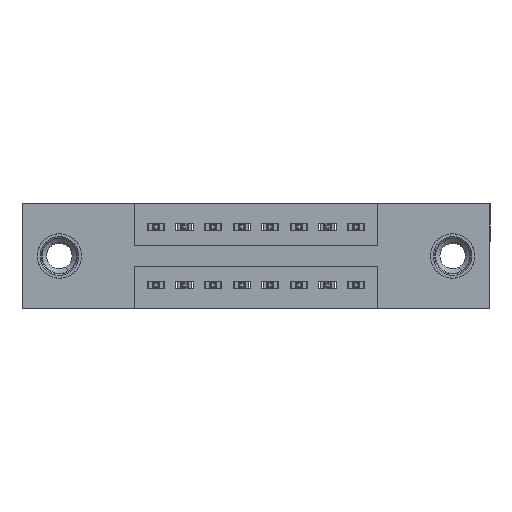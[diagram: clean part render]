
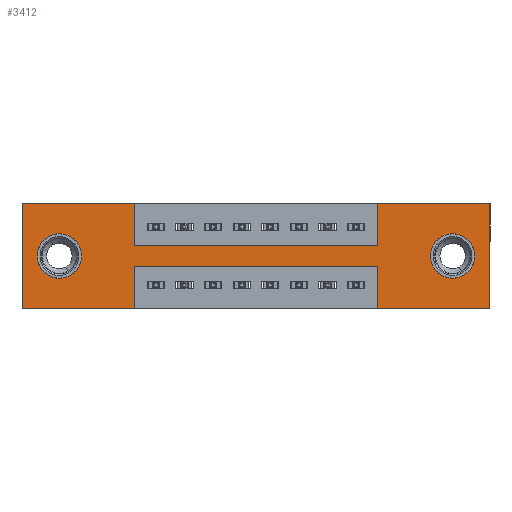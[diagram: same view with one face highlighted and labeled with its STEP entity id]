
A CAD part, front view. The second image highlights one B-rep face of the part: STEP entity #3412.
In plain terms, the highlighted planar face has unit normal (0, -1, 0).
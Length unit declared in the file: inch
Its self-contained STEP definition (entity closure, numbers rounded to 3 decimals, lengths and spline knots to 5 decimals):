
#125 = ORIENTED_EDGE ( 'NONE', *, *, #7274, .F. ) ;
#274 = DIRECTION ( 'NONE',  ( 0., 0., -1. ) ) ;
#283 = VERTEX_POINT ( 'NONE', #14115 ) ;
#378 = CIRCLE ( 'NONE', #13085, 0.078 ) ;
#395 = ORIENTED_EDGE ( 'NONE', *, *, #14176, .F. ) ;
#463 = CARTESIAN_POINT ( 'NONE',  ( 0., 0., -0.37 ) ) ;
#884 = EDGE_CURVE ( 'NONE', #5470, #13714, #1050, .T. ) ;
#1050 = LINE ( 'NONE', #11001, #4353 ) ;
#1182 = DIRECTION ( 'NONE',  ( -1., 0., 0. ) ) ;
#1227 = LINE ( 'NONE', #4448, #13803 ) ;
#1236 = VERTEX_POINT ( 'NONE', #10973 ) ;
#1474 = ORIENTED_EDGE ( 'NONE', *, *, #1575, .F. ) ;
#1477 = EDGE_CURVE ( 'NONE', #2456, #7086, #11795, .T. ) ;
#1521 = EDGE_CURVE ( 'NONE', #2381, #9207, #1227, .T. ) ;
#1575 = EDGE_CURVE ( 'NONE', #283, #8179, #10267, .T. ) ;
#1615 = PLANE ( 'NONE',  #13128 ) ;
#1668 = DIRECTION ( 'NONE',  ( 0., -1., 0. ) ) ;
#2303 = ORIENTED_EDGE ( 'NONE', *, *, #884, .F. ) ;
#2381 = VERTEX_POINT ( 'NONE', #4480 ) ;
#2395 = LINE ( 'NONE', #6970, #15334 ) ;
#2439 = VERTEX_POINT ( 'NONE', #3360 ) ;
#2456 = VERTEX_POINT ( 'NONE', #8356 ) ;
#3083 = AXIS2_PLACEMENT_3D ( 'NONE', #10974, #3603, #12173 ) ;
#3088 = CARTESIAN_POINT ( 'NONE',  ( 0., 0., -0.37 ) ) ;
#3190 = DIRECTION ( 'NONE',  ( -1., 0., 0. ) ) ;
#3360 = CARTESIAN_POINT ( 'NONE',  ( 0.13, 0., -0.107 ) ) ;
#3412 = ADVANCED_FACE ( 'NONE', ( #14576, #5364, #11462 ), #1615, .T. ) ;
#3509 = ORIENTED_EDGE ( 'NONE', *, *, #9941, .F. ) ;
#3603 = DIRECTION ( 'NONE',  ( 0., 1., 0. ) ) ;
#3614 = VERTEX_POINT ( 'NONE', #11869 ) ;
#3825 = DIRECTION ( 'NONE',  ( -1., 0., 0. ) ) ;
#3841 = ORIENTED_EDGE ( 'NONE', *, *, #14160, .F. ) ;
#4153 = DIRECTION ( 'NONE',  ( 1., 0., 0. ) ) ;
#4353 = VECTOR ( 'NONE', #10106, 39.37008 ) ;
#4409 = DIRECTION ( 'NONE',  ( 0., 1., 0. ) ) ;
#4448 = CARTESIAN_POINT ( 'NONE',  ( 0.3925, 0., -0.15 ) ) ;
#4460 = CIRCLE ( 'NONE', #8873, 0.078 ) ;
#4480 = CARTESIAN_POINT ( 'NONE',  ( 0.3925, 0., -0.15 ) ) ;
#4507 = DIRECTION ( 'NONE',  ( 0., 0., 1. ) ) ;
#4661 = LINE ( 'NONE', #12992, #10787 ) ;
#4708 = LINE ( 'NONE', #11189, #5100 ) ;
#4709 = ORIENTED_EDGE ( 'NONE', *, *, #8935, .T. ) ;
#4777 = DIRECTION ( 'NONE',  ( 1., 0., 0. ) ) ;
#4885 = CARTESIAN_POINT ( 'NONE',  ( 0., 0., 0. ) ) ;
#4926 = VECTOR ( 'NONE', #6058, 39.37008 ) ;
#5026 = ORIENTED_EDGE ( 'NONE', *, *, #9549, .T. ) ;
#5100 = VECTOR ( 'NONE', #3825, 39.37008 ) ;
#5149 = DIRECTION ( 'NONE',  ( 0., 0., -1. ) ) ;
#5195 = CARTESIAN_POINT ( 'NONE',  ( 1.2425, 0., -0.37 ) ) ;
#5274 = EDGE_LOOP ( 'NONE', ( #4709, #5026 ) ) ;
#5275 = VERTEX_POINT ( 'NONE', #10652 ) ;
#5364 = FACE_BOUND ( 'NONE', #5274, .T. ) ;
#5470 = VERTEX_POINT ( 'NONE', #7477 ) ;
#5484 = DIRECTION ( 'NONE',  ( 0., 1., 0. ) ) ;
#5611 = DIRECTION ( 'NONE',  ( 0., 0., 1. ) ) ;
#5828 = VECTOR ( 'NONE', #5611, 39.37008 ) ;
#5867 = VERTEX_POINT ( 'NONE', #14406 ) ;
#5991 = CARTESIAN_POINT ( 'NONE',  ( 0.3925, 0., 0. ) ) ;
#6058 = DIRECTION ( 'NONE',  ( 0., 0., -1. ) ) ;
#6106 = ORIENTED_EDGE ( 'NONE', *, *, #12078, .F. ) ;
#6606 = VECTOR ( 'NONE', #5149, 39.37008 ) ;
#6831 = CARTESIAN_POINT ( 'NONE',  ( 0., 0., 0. ) ) ;
#6970 = CARTESIAN_POINT ( 'NONE',  ( 1.635, 0., 0. ) ) ;
#7086 = VERTEX_POINT ( 'NONE', #12065 ) ;
#7274 = EDGE_CURVE ( 'NONE', #13714, #2381, #13028, .T. ) ;
#7325 = CARTESIAN_POINT ( 'NONE',  ( 0.3925, 0., -0.22 ) ) ;
#7390 = CARTESIAN_POINT ( 'NONE',  ( 1.2425, 0., -0.15 ) ) ;
#7445 = VECTOR ( 'NONE', #3190, 39.37008 ) ;
#7477 = CARTESIAN_POINT ( 'NONE',  ( 0., 0., 0. ) ) ;
#7574 = CARTESIAN_POINT ( 'NONE',  ( 0.3925, 0., 0. ) ) ;
#7671 = DIRECTION ( 'NONE',  ( 0., 1., 0. ) ) ;
#7842 = EDGE_LOOP ( 'NONE', ( #13222, #15052 ) ) ;
#8165 = EDGE_CURVE ( 'NONE', #5275, #3614, #4460, .T. ) ;
#8179 = VERTEX_POINT ( 'NONE', #5195 ) ;
#8316 = VERTEX_POINT ( 'NONE', #15069 ) ;
#8356 = CARTESIAN_POINT ( 'NONE',  ( 1.2425, 0., 0. ) ) ;
#8682 = ORIENTED_EDGE ( 'NONE', *, *, #1521, .F. ) ;
#8704 = LINE ( 'NONE', #6831, #14655 ) ;
#8873 = AXIS2_PLACEMENT_3D ( 'NONE', #14813, #7671, #274 ) ;
#8935 = EDGE_CURVE ( 'NONE', #2439, #5867, #378, .T. ) ;
#9023 = ORIENTED_EDGE ( 'NONE', *, *, #10426, .F. ) ;
#9207 = VERTEX_POINT ( 'NONE', #7390 ) ;
#9389 = EDGE_LOOP ( 'NONE', ( #6106, #13473, #13769, #1474, #9023, #11805, #3841, #8682, #125, #2303, #395, #3509 ) ) ;
#9549 = EDGE_CURVE ( 'NONE', #5867, #2439, #11117, .T. ) ;
#9645 = AXIS2_PLACEMENT_3D ( 'NONE', #12731, #5484, #13913 ) ;
#9781 = CARTESIAN_POINT ( 'NONE',  ( 0., 0., -0.37 ) ) ;
#9941 = EDGE_CURVE ( 'NONE', #1236, #8316, #15704, .T. ) ;
#10106 = DIRECTION ( 'NONE',  ( 1., 0., 0. ) ) ;
#10225 = CARTESIAN_POINT ( 'NONE',  ( 1.2425, 0., -0.22 ) ) ;
#10267 = LINE ( 'NONE', #3088, #7445 ) ;
#10282 = DIRECTION ( 'NONE',  ( 0., 0., -1. ) ) ;
#10426 = EDGE_CURVE ( 'NONE', #7086, #283, #2395, .T. ) ;
#10652 = CARTESIAN_POINT ( 'NONE',  ( 1.505, 0., -0.263 ) ) ;
#10787 = VECTOR ( 'NONE', #4507, 39.37008 ) ;
#10973 = CARTESIAN_POINT ( 'NONE',  ( 0.3925, 0., -0.37 ) ) ;
#10974 = CARTESIAN_POINT ( 'NONE',  ( 1.505, 0., -0.185 ) ) ;
#11001 = CARTESIAN_POINT ( 'NONE',  ( 0., 0., 0. ) ) ;
#11043 = LINE ( 'NONE', #13293, #4926 ) ;
#11117 = CIRCLE ( 'NONE', #9645, 0.078 ) ;
#11144 = VERTEX_POINT ( 'NONE', #10225 ) ;
#11189 = CARTESIAN_POINT ( 'NONE',  ( 0.3925, 0., -0.22 ) ) ;
#11462 = FACE_OUTER_BOUND ( 'NONE', #9389, .T. ) ;
#11526 = VERTEX_POINT ( 'NONE', #7325 ) ;
#11738 = CARTESIAN_POINT ( 'NONE',  ( 0.13, 0., -0.185 ) ) ;
#11795 = LINE ( 'NONE', #4885, #14535 ) ;
#11805 = ORIENTED_EDGE ( 'NONE', *, *, #1477, .F. ) ;
#11869 = CARTESIAN_POINT ( 'NONE',  ( 1.505, 0., -0.107 ) ) ;
#12065 = CARTESIAN_POINT ( 'NONE',  ( 1.635, 0., 0. ) ) ;
#12078 = EDGE_CURVE ( 'NONE', #11526, #1236, #11043, .T. ) ;
#12173 = DIRECTION ( 'NONE',  ( 0., 0., -1. ) ) ;
#12731 = CARTESIAN_POINT ( 'NONE',  ( 0.13, 0., -0.185 ) ) ;
#12767 = EDGE_CURVE ( 'NONE', #11144, #11526, #4708, .T. ) ;
#12840 = CARTESIAN_POINT ( 'NONE',  ( 1.2425, 0., 0. ) ) ;
#12898 = DIRECTION ( 'NONE',  ( 0., 0., 1. ) ) ;
#12992 = CARTESIAN_POINT ( 'NONE',  ( 1.2425, 0., -0.37 ) ) ;
#13028 = LINE ( 'NONE', #7574, #6606 ) ;
#13085 = AXIS2_PLACEMENT_3D ( 'NONE', #11738, #4409, #12898 ) ;
#13128 = AXIS2_PLACEMENT_3D ( 'NONE', #463, #1668, #10282 ) ;
#13222 = ORIENTED_EDGE ( 'NONE', *, *, #14456, .T. ) ;
#13293 = CARTESIAN_POINT ( 'NONE',  ( 0.3925, 0., -0.37 ) ) ;
#13473 = ORIENTED_EDGE ( 'NONE', *, *, #12767, .F. ) ;
#13714 = VERTEX_POINT ( 'NONE', #5991 ) ;
#13769 = ORIENTED_EDGE ( 'NONE', *, *, #14245, .F. ) ;
#13803 = VECTOR ( 'NONE', #4153, 39.37008 ) ;
#13913 = DIRECTION ( 'NONE',  ( 0., 0., 1. ) ) ;
#14019 = DIRECTION ( 'NONE',  ( 0., 0., 1. ) ) ;
#14103 = CIRCLE ( 'NONE', #3083, 0.078 ) ;
#14115 = CARTESIAN_POINT ( 'NONE',  ( 1.635, 0., -0.37 ) ) ;
#14160 = EDGE_CURVE ( 'NONE', #9207, #2456, #15029, .T. ) ;
#14176 = EDGE_CURVE ( 'NONE', #8316, #5470, #8704, .T. ) ;
#14245 = EDGE_CURVE ( 'NONE', #8179, #11144, #4661, .T. ) ;
#14406 = CARTESIAN_POINT ( 'NONE',  ( 0.13, 0., -0.263 ) ) ;
#14456 = EDGE_CURVE ( 'NONE', #3614, #5275, #14103, .T. ) ;
#14535 = VECTOR ( 'NONE', #4777, 39.37008 ) ;
#14576 = FACE_BOUND ( 'NONE', #7842, .T. ) ;
#14655 = VECTOR ( 'NONE', #14019, 39.37008 ) ;
#14813 = CARTESIAN_POINT ( 'NONE',  ( 1.505, 0., -0.185 ) ) ;
#14964 = VECTOR ( 'NONE', #1182, 39.37008 ) ;
#15029 = LINE ( 'NONE', #12840, #5828 ) ;
#15052 = ORIENTED_EDGE ( 'NONE', *, *, #8165, .T. ) ;
#15069 = CARTESIAN_POINT ( 'NONE',  ( 0., 0., -0.37 ) ) ;
#15334 = VECTOR ( 'NONE', #15339, 39.37008 ) ;
#15339 = DIRECTION ( 'NONE',  ( 0., 0., -1. ) ) ;
#15704 = LINE ( 'NONE', #9781, #14964 ) ;
